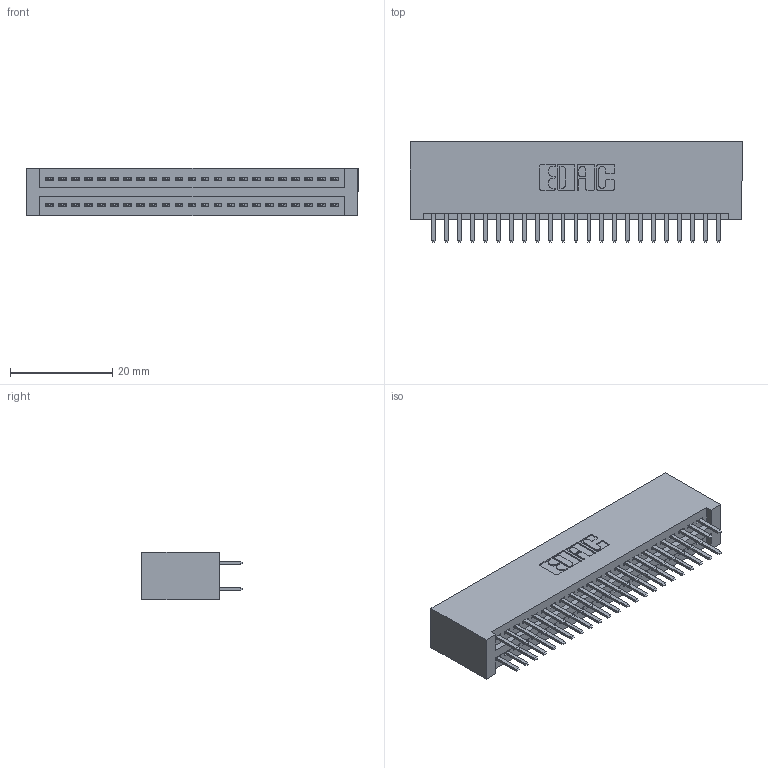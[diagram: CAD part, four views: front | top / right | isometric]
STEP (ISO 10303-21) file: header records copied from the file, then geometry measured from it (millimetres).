
FILE_DESCRIPTION (( 'STEP AP203' ), '1' );
FILE_NAME ('395-046-520-201.STEP', '2019-10-19T03:21:12', ( '' ), ( '' ), 'SwSTEP 2.0', 'SolidWorks 2016', '' );
FILE_SCHEMA (( 'CONFIG_CONTROL_DESIGN' ));
Length unit declared in the file: inch
Products named in the file (3): 345 Part_No Mounting Lugs; 345-292-001_345-293-120; 395-046-520-201
Assembly tree (47 placements, depth 2):
  395-046-520-201
    345 Part_No Mounting Lugs
    345-292-001_345-293-120  x46
Bounding box: 65.02 x 19.68 x 9.4 mm (x, y, z)
Volume: 6735.8 mm3; surface area: 9848.9 mm2
Topology: 47 solids, 47 shells, 2602 faces, 7539 edges, 4902 vertices
Faces by surface type: plane 1686, cylinder 916
Entity records: 20441 total; most frequent: CARTESIAN_POINT 3456, ORIENTED_EDGE 3378, DIRECTION 3053, EDGE_CURVE 1689, VECTOR 1469, LINE 1469, VERTEX_POINT 1122, AXIS2_PLACEMENT_3D 792
